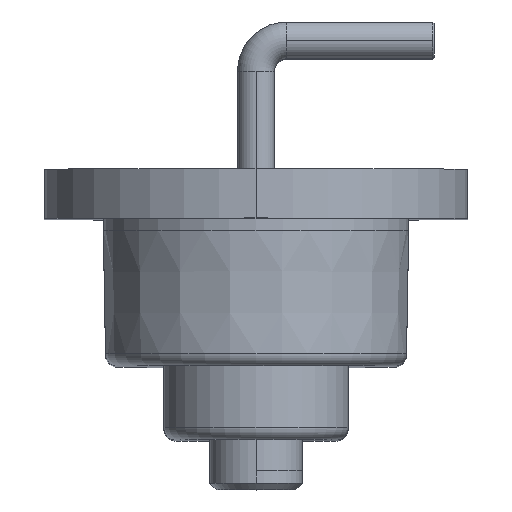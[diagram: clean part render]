
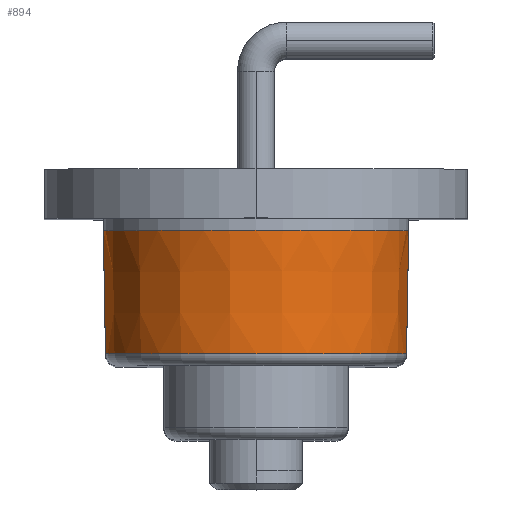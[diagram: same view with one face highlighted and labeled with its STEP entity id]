
A CAD part, top view. The second image highlights one B-rep face of the part: STEP entity #894.
In plain terms, the highlighted conical face has half-angle 1 degrees and reference radius 2.465 mm.
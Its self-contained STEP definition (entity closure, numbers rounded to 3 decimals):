
#321 = VERTEX_POINT ( 'NONE', #7327 ) ;
#430 = LINE ( 'NONE', #2750, #613 ) ;
#583 = CONICAL_SURFACE ( 'NONE', #4108, 2.465, 0.017 ) ;
#613 = VECTOR ( 'NONE', #2053, 1000. ) ;
#894 = ADVANCED_FACE ( 'NONE', ( #5753 ), #583, .T. ) ;
#922 = ORIENTED_EDGE ( 'NONE', *, *, #2247, .F. ) ;
#996 = ORIENTED_EDGE ( 'NONE', *, *, #2212, .T. ) ;
#1008 = VERTEX_POINT ( 'NONE', #6647 ) ;
#1031 = VERTEX_POINT ( 'NONE', #7338 ) ;
#1192 = EDGE_LOOP ( 'NONE', ( #3224, #922, #2154, #996 ) ) ;
#1717 = CARTESIAN_POINT ( 'NONE',  ( -2.448, 22.937, 6.5 ) ) ;
#1836 = DIRECTION ( 'NONE',  ( -1., 0., 0.019 ) ) ;
#2053 = DIRECTION ( 'NONE',  ( -0.017, -1., 0. ) ) ;
#2154 = ORIENTED_EDGE ( 'NONE', *, *, #6984, .F. ) ;
#2212 = EDGE_CURVE ( 'NONE', #4030, #1008, #7491, .T. ) ;
#2247 = EDGE_CURVE ( 'NONE', #1031, #321, #3137, .T. ) ;
#2364 = LINE ( 'NONE', #1717, #6800 ) ;
#2365 = DIRECTION ( 'NONE',  ( -1., 0., 0. ) ) ;
#2392 = AXIS2_PLACEMENT_3D ( 'NONE', #3595, #2553, #1836 ) ;
#2446 = DIRECTION ( 'NONE',  ( -1., 0., 0. ) ) ;
#2553 = DIRECTION ( 'NONE',  ( 0., 1., 0. ) ) ;
#2750 = CARTESIAN_POINT ( 'NONE',  ( 2.483, 24.94, 6.5 ) ) ;
#3092 = DIRECTION ( 'NONE',  ( 0., 1., 0. ) ) ;
#3137 = CIRCLE ( 'NONE', #3385, 2.483 ) ;
#3224 = ORIENTED_EDGE ( 'NONE', *, *, #7212, .F. ) ;
#3385 = AXIS2_PLACEMENT_3D ( 'NONE', #5866, #3092, #2446 ) ;
#3558 = DIRECTION ( 'NONE',  ( 0., 1., 0. ) ) ;
#3595 = CARTESIAN_POINT ( 'NONE',  ( 0., 22.937, 6.5 ) ) ;
#4030 = VERTEX_POINT ( 'NONE', #4132 ) ;
#4108 = AXIS2_PLACEMENT_3D ( 'NONE', #4163, #3558, #2365 ) ;
#4132 = CARTESIAN_POINT ( 'NONE',  ( -2.448, 22.937, 6.5 ) ) ;
#4163 = CARTESIAN_POINT ( 'NONE',  ( 0., 23.938, 6.5 ) ) ;
#5753 = FACE_OUTER_BOUND ( 'NONE', #1192, .T. ) ;
#5866 = CARTESIAN_POINT ( 'NONE',  ( 0., 24.94, 6.5 ) ) ;
#6356 = DIRECTION ( 'NONE',  ( -0.017, 1., 0. ) ) ;
#6647 = CARTESIAN_POINT ( 'NONE',  ( 2.448, 22.937, 6.5 ) ) ;
#6800 = VECTOR ( 'NONE', #6356, 1000. ) ;
#6984 = EDGE_CURVE ( 'NONE', #4030, #1031, #2364, .T. ) ;
#7212 = EDGE_CURVE ( 'NONE', #321, #1008, #430, .T. ) ;
#7327 = CARTESIAN_POINT ( 'NONE',  ( 2.483, 24.94, 6.5 ) ) ;
#7338 = CARTESIAN_POINT ( 'NONE',  ( -2.483, 24.94, 6.5 ) ) ;
#7491 = CIRCLE ( 'NONE', #2392, 2.448 ) ;
